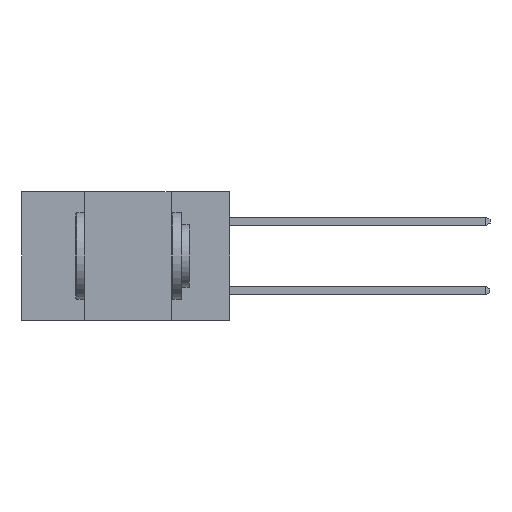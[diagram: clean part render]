
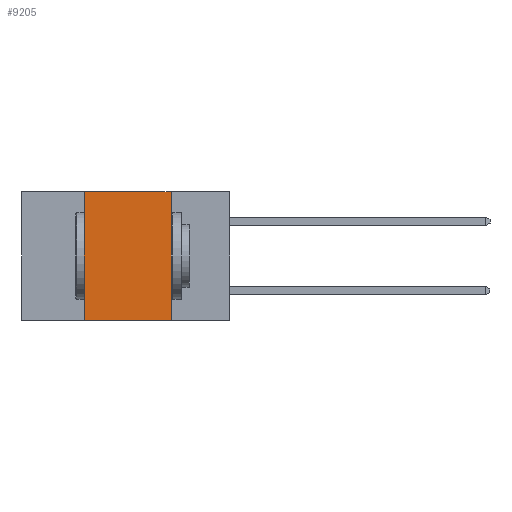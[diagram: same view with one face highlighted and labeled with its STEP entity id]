
A CAD part, left-side view. The second image highlights one B-rep face of the part: STEP entity #9205.
In plain terms, the highlighted planar face has unit normal (-1, 0, 0).
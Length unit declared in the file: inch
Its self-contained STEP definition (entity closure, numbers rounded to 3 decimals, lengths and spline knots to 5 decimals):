
#221 = DIRECTION ( 'NONE',  ( 0., 0., -1. ) ) ;
#449 = VERTEX_POINT ( 'NONE', #22995 ) ;
#668 = FACE_OUTER_BOUND ( 'NONE', #11611, .T. ) ;
#823 = DIRECTION ( 'NONE',  ( 0., 0., 1. ) ) ;
#892 = VECTOR ( 'NONE', #823, 39.37008 ) ;
#1233 = CARTESIAN_POINT ( 'NONE',  ( 0., 0.42, -0.37 ) ) ;
#1418 = CARTESIAN_POINT ( 'NONE',  ( 0., 0.17, 0. ) ) ;
#1606 = LINE ( 'NONE', #1418, #14337 ) ;
#1630 = LINE ( 'NONE', #24190, #892 ) ;
#4394 = AXIS2_PLACEMENT_3D ( 'NONE', #7387, #14545, #221 ) ;
#5631 = ORIENTED_EDGE ( 'NONE', *, *, #23122, .F. ) ;
#6274 = DIRECTION ( 'NONE',  ( 0., 0., -1. ) ) ;
#7099 = DIRECTION ( 'NONE',  ( 0., -1., 0. ) ) ;
#7387 = CARTESIAN_POINT ( 'NONE',  ( 0., 0.6, 0. ) ) ;
#8535 = CARTESIAN_POINT ( 'NONE',  ( 0., 0.17, 0. ) ) ;
#8717 = VECTOR ( 'NONE', #15720, 39.37008 ) ;
#9038 = LINE ( 'NONE', #13504, #8717 ) ;
#9205 = ADVANCED_FACE ( 'NONE', ( #668 ), #28212, .F. ) ;
#10459 = ORIENTED_EDGE ( 'NONE', *, *, #28469, .F. ) ;
#11477 = VERTEX_POINT ( 'NONE', #8535 ) ;
#11611 = EDGE_LOOP ( 'NONE', ( #28103, #10459, #5631, #18198 ) ) ;
#12801 = EDGE_CURVE ( 'NONE', #11477, #29886, #1606, .T. ) ;
#13504 = CARTESIAN_POINT ( 'NONE',  ( 0., 0.6, -0.37 ) ) ;
#14337 = VECTOR ( 'NONE', #6274, 39.37008 ) ;
#14545 = DIRECTION ( 'NONE',  ( 1., 0., 0. ) ) ;
#15720 = DIRECTION ( 'NONE',  ( 0., -1., 0. ) ) ;
#16251 = VECTOR ( 'NONE', #7099, 39.37008 ) ;
#18198 = ORIENTED_EDGE ( 'NONE', *, *, #25532, .T. ) ;
#19505 = CARTESIAN_POINT ( 'NONE',  ( 0., 0.17, -0.37 ) ) ;
#21198 = CARTESIAN_POINT ( 'NONE',  ( 0., 0.6, 0. ) ) ;
#21734 = LINE ( 'NONE', #21198, #16251 ) ;
#22995 = CARTESIAN_POINT ( 'NONE',  ( 0., 0.42, 0. ) ) ;
#23122 = EDGE_CURVE ( 'NONE', #25488, #449, #1630, .T. ) ;
#24190 = CARTESIAN_POINT ( 'NONE',  ( 0., 0.42, 0. ) ) ;
#25488 = VERTEX_POINT ( 'NONE', #1233 ) ;
#25532 = EDGE_CURVE ( 'NONE', #25488, #29886, #9038, .T. ) ;
#28103 = ORIENTED_EDGE ( 'NONE', *, *, #12801, .F. ) ;
#28212 = PLANE ( 'NONE',  #4394 ) ;
#28469 = EDGE_CURVE ( 'NONE', #449, #11477, #21734, .T. ) ;
#29886 = VERTEX_POINT ( 'NONE', #19505 ) ;
